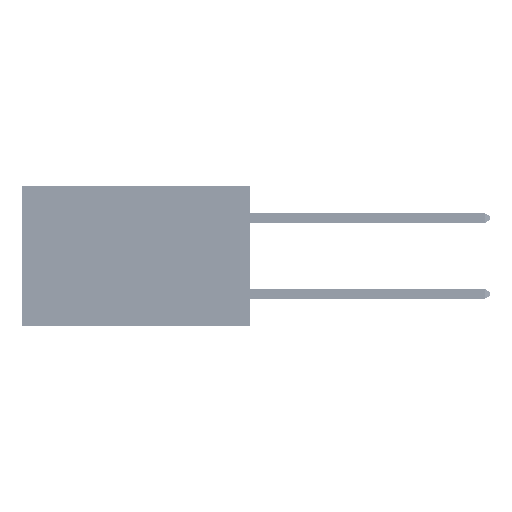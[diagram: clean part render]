
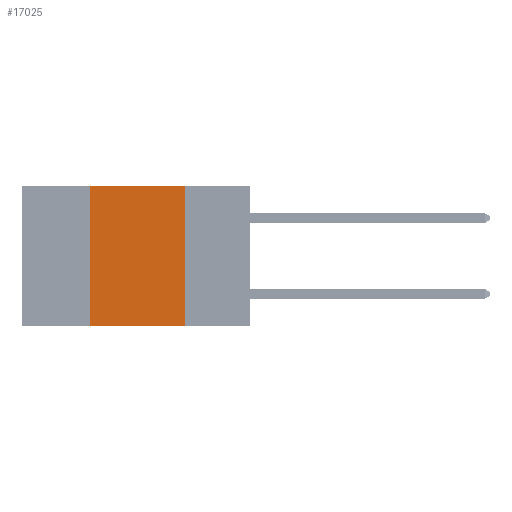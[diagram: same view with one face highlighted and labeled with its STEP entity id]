
A CAD part, left-side view. The second image highlights one B-rep face of the part: STEP entity #17025.
In plain terms, the highlighted planar face has unit normal (-1, 0, 0).
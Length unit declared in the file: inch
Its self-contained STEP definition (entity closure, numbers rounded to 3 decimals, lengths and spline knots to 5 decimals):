
#3374 = VECTOR ( 'NONE', #13559, 39.37008 ) ;
#4473 = VECTOR ( 'NONE', #13280, 39.37008 ) ;
#5593 = CARTESIAN_POINT ( 'NONE',  ( 0., 0.17, 0. ) ) ;
#5707 = CARTESIAN_POINT ( 'NONE',  ( 0., 0.6, -0.37 ) ) ;
#5831 = DIRECTION ( 'NONE',  ( 0., 0., 1. ) ) ;
#7156 = CARTESIAN_POINT ( 'NONE',  ( 0., 0.6, 0. ) ) ;
#7917 = CARTESIAN_POINT ( 'NONE',  ( 0., 0.17, -0.37 ) ) ;
#8149 = VERTEX_POINT ( 'NONE', #16250 ) ;
#11116 = ORIENTED_EDGE ( 'NONE', *, *, #39271, .F. ) ;
#13280 = DIRECTION ( 'NONE',  ( 0., 0., -1. ) ) ;
#13559 = DIRECTION ( 'NONE',  ( 0., -1., 0. ) ) ;
#13679 = CARTESIAN_POINT ( 'NONE',  ( 0., 0.42, 0. ) ) ;
#16250 = CARTESIAN_POINT ( 'NONE',  ( 0., 0.42, -0.37 ) ) ;
#16643 = ORIENTED_EDGE ( 'NONE', *, *, #18774, .F. ) ;
#17025 = ADVANCED_FACE ( 'NONE', ( #40887 ), #42147, .F. ) ;
#17425 = EDGE_CURVE ( 'NONE', #8149, #25222, #24139, .T. ) ;
#18774 = EDGE_CURVE ( 'NONE', #35885, #25222, #45425, .T. ) ;
#19285 = AXIS2_PLACEMENT_3D ( 'NONE', #23129, #49718, #26931 ) ;
#20335 = ORIENTED_EDGE ( 'NONE', *, *, #46081, .F. ) ;
#21953 = LINE ( 'NONE', #7156, #29657 ) ;
#23129 = CARTESIAN_POINT ( 'NONE',  ( 0., 0.6, 0. ) ) ;
#24004 = VERTEX_POINT ( 'NONE', #31479 ) ;
#24139 = LINE ( 'NONE', #5707, #3374 ) ;
#25222 = VERTEX_POINT ( 'NONE', #7917 ) ;
#26931 = DIRECTION ( 'NONE',  ( 0., 0., -1. ) ) ;
#29358 = CARTESIAN_POINT ( 'NONE',  ( 0., 0.17, 0. ) ) ;
#29657 = VECTOR ( 'NONE', #38003, 39.37008 ) ;
#29863 = LINE ( 'NONE', #13679, #38869 ) ;
#31479 = CARTESIAN_POINT ( 'NONE',  ( 0., 0.42, 0. ) ) ;
#35885 = VERTEX_POINT ( 'NONE', #29358 ) ;
#38003 = DIRECTION ( 'NONE',  ( 0., -1., 0. ) ) ;
#38869 = VECTOR ( 'NONE', #5831, 39.37008 ) ;
#39271 = EDGE_CURVE ( 'NONE', #8149, #24004, #29863, .T. ) ;
#40887 = FACE_OUTER_BOUND ( 'NONE', #42889, .T. ) ;
#42147 = PLANE ( 'NONE',  #19285 ) ;
#42889 = EDGE_LOOP ( 'NONE', ( #16643, #20335, #11116, #44174 ) ) ;
#44174 = ORIENTED_EDGE ( 'NONE', *, *, #17425, .T. ) ;
#45425 = LINE ( 'NONE', #5593, #4473 ) ;
#46081 = EDGE_CURVE ( 'NONE', #24004, #35885, #21953, .T. ) ;
#49718 = DIRECTION ( 'NONE',  ( 1., 0., 0. ) ) ;
